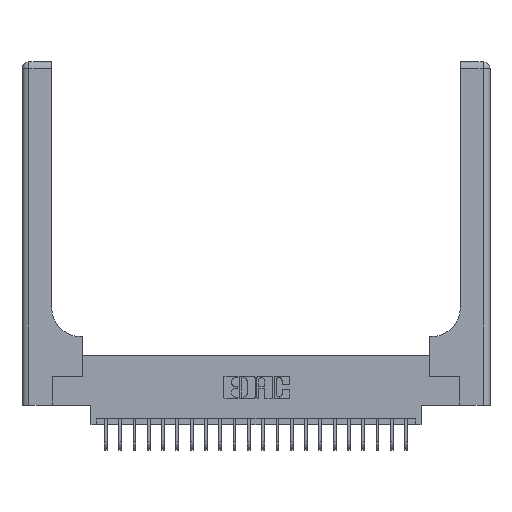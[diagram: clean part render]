
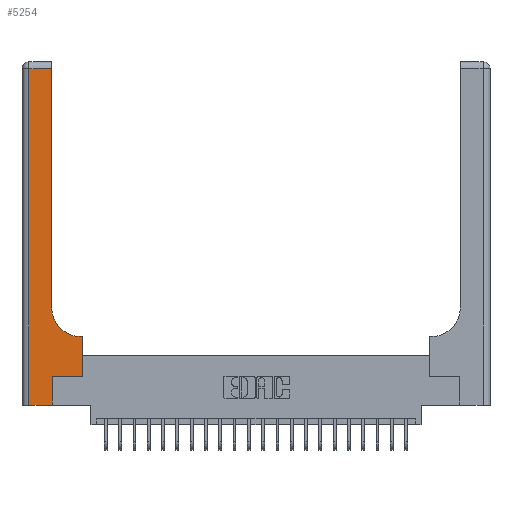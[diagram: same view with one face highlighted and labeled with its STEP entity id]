
A CAD part, top view. The second image highlights one B-rep face of the part: STEP entity #5254.
In plain terms, the highlighted planar face has unit normal (0, 0, 1).
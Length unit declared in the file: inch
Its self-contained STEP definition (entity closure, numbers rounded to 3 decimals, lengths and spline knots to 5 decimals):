
#149 = VECTOR ( 'NONE', #23073, 39.37008 ) ;
#503 = LINE ( 'NONE', #1657, #6324 ) ;
#675 = CARTESIAN_POINT ( 'NONE',  ( 0.51, 0.85, 0.37 ) ) ;
#1657 = CARTESIAN_POINT ( 'NONE',  ( 0., 0., 0.37 ) ) ;
#1979 = DIRECTION ( 'NONE',  ( 0., -1., 0. ) ) ;
#2014 = VERTEX_POINT ( 'NONE', #11019 ) ;
#2114 = DIRECTION ( 'NONE',  ( 1., 0., 0. ) ) ;
#2879 = DIRECTION ( 'NONE',  ( -1., 0., 0. ) ) ;
#3846 = VERTEX_POINT ( 'NONE', #21373 ) ;
#4488 = EDGE_CURVE ( 'NONE', #2014, #21023, #12259, .T. ) ;
#4816 = CARTESIAN_POINT ( 'NONE',  ( 0.528, 0.25, 0.37 ) ) ;
#4858 = DIRECTION ( 'NONE',  ( 0., 1., 0. ) ) ;
#5254 = ADVANCED_FACE ( 'NONE', ( #14870 ), #12386, .F. ) ;
#5443 = VERTEX_POINT ( 'NONE', #21426 ) ;
#5881 = AXIS2_PLACEMENT_3D ( 'NONE', #675, #13692, #11977 ) ;
#6040 = VECTOR ( 'NONE', #2879, 39.37008 ) ;
#6134 = CARTESIAN_POINT ( 'NONE',  ( 0.265, 0., 0.37 ) ) ;
#6324 = VECTOR ( 'NONE', #9084, 39.37008 ) ;
#6393 = EDGE_CURVE ( 'NONE', #10463, #8921, #20075, .T. ) ;
#6514 = CARTESIAN_POINT ( 'NONE',  ( 0.265, 0., 0.37 ) ) ;
#6576 = VERTEX_POINT ( 'NONE', #10113 ) ;
#7046 = ORIENTED_EDGE ( 'NONE', *, *, #10904, .T. ) ;
#7982 = EDGE_CURVE ( 'NONE', #8921, #19620, #8048, .T. ) ;
#8048 = LINE ( 'NONE', #21155, #149 ) ;
#8921 = VERTEX_POINT ( 'NONE', #4816 ) ;
#9084 = DIRECTION ( 'NONE',  ( 1., 0., 0. ) ) ;
#9292 = LINE ( 'NONE', #15716, #6040 ) ;
#9512 = VECTOR ( 'NONE', #17389, 39.37008 ) ;
#10113 = CARTESIAN_POINT ( 'NONE',  ( 0.51, 0.6, 0.37 ) ) ;
#10126 = CARTESIAN_POINT ( 'NONE',  ( 0., 2.94, 0.37 ) ) ;
#10463 = VERTEX_POINT ( 'NONE', #18291 ) ;
#10695 = DIRECTION ( 'NONE',  ( -1., 0., 0. ) ) ;
#10904 = EDGE_CURVE ( 'NONE', #6576, #3846, #20487, .T. ) ;
#11019 = CARTESIAN_POINT ( 'NONE',  ( 0.26, 2.94, 0.37 ) ) ;
#11036 = LINE ( 'NONE', #6514, #19225 ) ;
#11052 = CARTESIAN_POINT ( 'NONE',  ( 0.06, 3., 0.37 ) ) ;
#11117 = VECTOR ( 'NONE', #19533, 39.37008 ) ;
#11977 = DIRECTION ( 'NONE',  ( 1., 0., 0. ) ) ;
#12123 = VECTOR ( 'NONE', #1979, 39.37008 ) ;
#12259 = LINE ( 'NONE', #10126, #11117 ) ;
#12386 = PLANE ( 'NONE',  #21468 ) ;
#13306 = LINE ( 'NONE', #11052, #12123 ) ;
#13692 = DIRECTION ( 'NONE',  ( 0., 0., -1. ) ) ;
#13918 = ORIENTED_EDGE ( 'NONE', *, *, #7982, .T. ) ;
#13986 = ORIENTED_EDGE ( 'NONE', *, *, #4488, .T. ) ;
#14425 = DIRECTION ( 'NONE',  ( 0., 0., -1. ) ) ;
#14870 = FACE_OUTER_BOUND ( 'NONE', #16953, .T. ) ;
#14964 = EDGE_CURVE ( 'NONE', #17239, #10463, #11036, .T. ) ;
#14989 = EDGE_CURVE ( 'NONE', #19620, #6576, #9292, .T. ) ;
#15117 = ORIENTED_EDGE ( 'NONE', *, *, #14989, .T. ) ;
#15157 = ORIENTED_EDGE ( 'NONE', *, *, #14964, .T. ) ;
#15714 = EDGE_CURVE ( 'NONE', #5443, #17239, #503, .T. ) ;
#15716 = CARTESIAN_POINT ( 'NONE',  ( 0.26, 0.6, 0.37 ) ) ;
#15798 = ORIENTED_EDGE ( 'NONE', *, *, #23036, .T. ) ;
#16185 = EDGE_CURVE ( 'NONE', #21023, #5443, #13306, .T. ) ;
#16811 = LINE ( 'NONE', #17138, #9512 ) ;
#16953 = EDGE_LOOP ( 'NONE', ( #15798, #13986, #17443, #16956, #15157, #19837, #13918, #15117, #7046 ) ) ;
#16956 = ORIENTED_EDGE ( 'NONE', *, *, #15714, .T. ) ;
#17138 = CARTESIAN_POINT ( 'NONE',  ( 0.26, 3., 0.37 ) ) ;
#17231 = CARTESIAN_POINT ( 'NONE',  ( 0.265, 0.25, 0.37 ) ) ;
#17239 = VERTEX_POINT ( 'NONE', #6134 ) ;
#17389 = DIRECTION ( 'NONE',  ( 0., 1., 0. ) ) ;
#17443 = ORIENTED_EDGE ( 'NONE', *, *, #16185, .T. ) ;
#17698 = CARTESIAN_POINT ( 'NONE',  ( 0.06, 2.94, 0.37 ) ) ;
#18291 = CARTESIAN_POINT ( 'NONE',  ( 0.265, 0.25, 0.37 ) ) ;
#19225 = VECTOR ( 'NONE', #4858, 39.37008 ) ;
#19533 = DIRECTION ( 'NONE',  ( -1., 0., 0. ) ) ;
#19620 = VERTEX_POINT ( 'NONE', #22590 ) ;
#19837 = ORIENTED_EDGE ( 'NONE', *, *, #6393, .T. ) ;
#20075 = LINE ( 'NONE', #17231, #20384 ) ;
#20384 = VECTOR ( 'NONE', #2114, 39.37008 ) ;
#20487 = CIRCLE ( 'NONE', #5881, 0.25 ) ;
#21023 = VERTEX_POINT ( 'NONE', #17698 ) ;
#21155 = CARTESIAN_POINT ( 'NONE',  ( 0.528, 0.25, 0.37 ) ) ;
#21373 = CARTESIAN_POINT ( 'NONE',  ( 0.26, 0.85, 0.37 ) ) ;
#21426 = CARTESIAN_POINT ( 'NONE',  ( 0.06, 0., 0.37 ) ) ;
#21468 = AXIS2_PLACEMENT_3D ( 'NONE', #21824, #14425, #10695 ) ;
#21824 = CARTESIAN_POINT ( 'NONE',  ( 0., 3., 0.37 ) ) ;
#22590 = CARTESIAN_POINT ( 'NONE',  ( 0.528, 0.6, 0.37 ) ) ;
#23036 = EDGE_CURVE ( 'NONE', #3846, #2014, #16811, .T. ) ;
#23073 = DIRECTION ( 'NONE',  ( 0., 1., 0. ) ) ;
